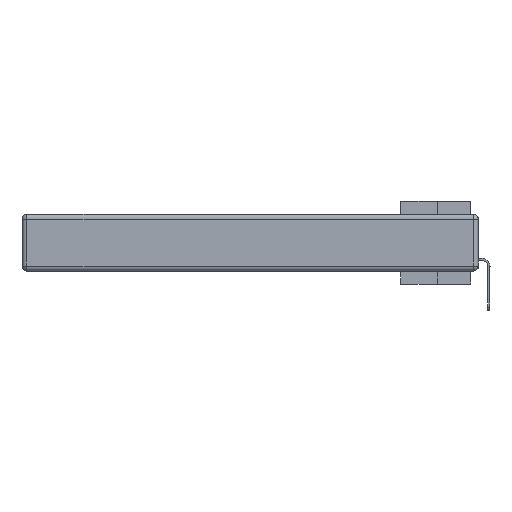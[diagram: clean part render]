
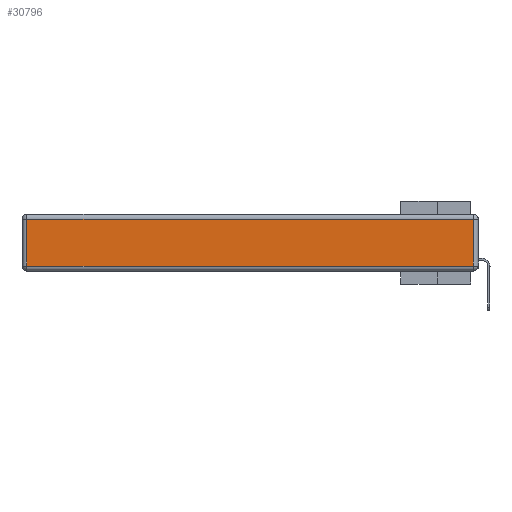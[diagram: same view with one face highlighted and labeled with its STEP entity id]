
A CAD part, left-side view. The second image highlights one B-rep face of the part: STEP entity #30796.
In plain terms, the highlighted planar face has unit normal (-1, 0, 0).
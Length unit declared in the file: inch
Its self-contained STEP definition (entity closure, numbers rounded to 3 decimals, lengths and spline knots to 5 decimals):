
#586 = DIRECTION ( 'NONE',  ( 0., 0., -1. ) ) ;
#1310 = VECTOR ( 'NONE', #23828, 39.37008 ) ;
#1902 = DIRECTION ( 'NONE',  ( 0., 0., 1. ) ) ;
#2363 = DIRECTION ( 'NONE',  ( 0., 0., 1. ) ) ;
#2538 = PLANE ( 'NONE',  #3923 ) ;
#2705 = LINE ( 'NONE', #14963, #15358 ) ;
#3226 = EDGE_CURVE ( 'NONE', #7665, #22875, #2705, .T. ) ;
#3923 = AXIS2_PLACEMENT_3D ( 'NONE', #24265, #7124, #1902 ) ;
#4074 = VERTEX_POINT ( 'NONE', #23028 ) ;
#6092 = ORIENTED_EDGE ( 'NONE', *, *, #3226, .T. ) ;
#6674 = CARTESIAN_POINT ( 'NONE',  ( 0., 2.75, -0.03 ) ) ;
#6899 = VECTOR ( 'NONE', #8688, 39.37008 ) ;
#7124 = DIRECTION ( 'NONE',  ( -1., 0., 0. ) ) ;
#7665 = VERTEX_POINT ( 'NONE', #8047 ) ;
#8047 = CARTESIAN_POINT ( 'NONE',  ( 0., 2.72, -0.03 ) ) ;
#8148 = VECTOR ( 'NONE', #2363, 39.37008 ) ;
#8688 = DIRECTION ( 'NONE',  ( 0., -1., 0. ) ) ;
#11918 = ORIENTED_EDGE ( 'NONE', *, *, #22759, .T. ) ;
#14963 = CARTESIAN_POINT ( 'NONE',  ( 0., 2.72, -0.343 ) ) ;
#15358 = VECTOR ( 'NONE', #586, 39.37008 ) ;
#17011 = CARTESIAN_POINT ( 'NONE',  ( 0., 2.72, -0.313 ) ) ;
#17218 = LINE ( 'NONE', #19670, #8148 ) ;
#19670 = CARTESIAN_POINT ( 'NONE',  ( 0., 0.03, -0.343 ) ) ;
#21104 = CARTESIAN_POINT ( 'NONE',  ( 0., 0., -0.313 ) ) ;
#22759 = EDGE_CURVE ( 'NONE', #22875, #26413, #29252, .T. ) ;
#22875 = VERTEX_POINT ( 'NONE', #17011 ) ;
#23028 = CARTESIAN_POINT ( 'NONE',  ( 0., 0.03, -0.03 ) ) ;
#23828 = DIRECTION ( 'NONE',  ( 0., 1., 0. ) ) ;
#24265 = CARTESIAN_POINT ( 'NONE',  ( 0., 0., -0.343 ) ) ;
#25478 = EDGE_LOOP ( 'NONE', ( #11918, #31916, #29265, #6092 ) ) ;
#26035 = EDGE_CURVE ( 'NONE', #26413, #4074, #17218, .T. ) ;
#26413 = VERTEX_POINT ( 'NONE', #31253 ) ;
#27198 = FACE_OUTER_BOUND ( 'NONE', #25478, .T. ) ;
#29063 = LINE ( 'NONE', #6674, #1310 ) ;
#29252 = LINE ( 'NONE', #21104, #6899 ) ;
#29265 = ORIENTED_EDGE ( 'NONE', *, *, #32135, .T. ) ;
#30796 = ADVANCED_FACE ( 'NONE', ( #27198 ), #2538, .T. ) ;
#31253 = CARTESIAN_POINT ( 'NONE',  ( 0., 0.03, -0.313 ) ) ;
#31916 = ORIENTED_EDGE ( 'NONE', *, *, #26035, .T. ) ;
#32135 = EDGE_CURVE ( 'NONE', #4074, #7665, #29063, .T. ) ;
